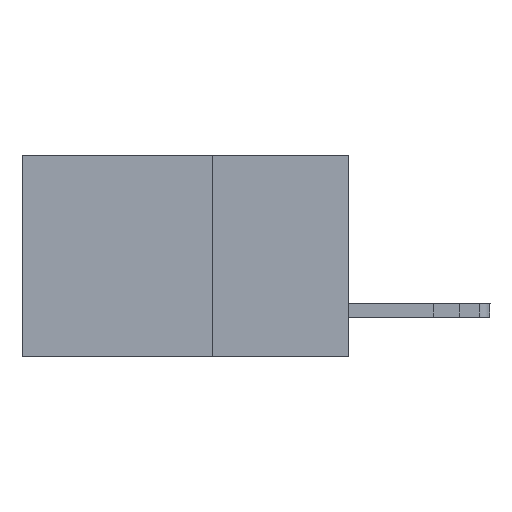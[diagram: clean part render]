
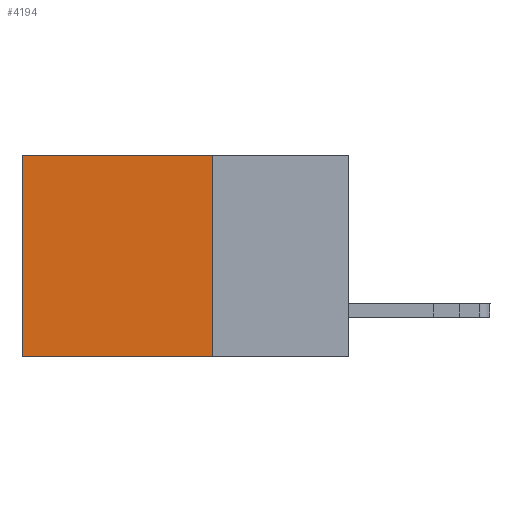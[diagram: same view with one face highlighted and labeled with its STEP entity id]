
A CAD part, left-side view. The second image highlights one B-rep face of the part: STEP entity #4194.
In plain terms, the highlighted planar face has unit normal (-1, 0, 0).
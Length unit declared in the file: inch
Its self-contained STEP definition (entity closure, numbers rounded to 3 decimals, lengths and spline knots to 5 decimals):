
#61 = ORIENTED_EDGE ( 'NONE', *, *, #4555, .F. ) ;
#358 = LINE ( 'NONE', #9970, #3960 ) ;
#395 = EDGE_CURVE ( 'NONE', #9664, #6442, #2372, .T. ) ;
#2223 = ORIENTED_EDGE ( 'NONE', *, *, #9491, .T. ) ;
#2327 = LINE ( 'NONE', #10978, #8749 ) ;
#2372 = LINE ( 'NONE', #5897, #4673 ) ;
#2373 = VERTEX_POINT ( 'NONE', #7644 ) ;
#2380 = VERTEX_POINT ( 'NONE', #3379 ) ;
#2879 = ORIENTED_EDGE ( 'NONE', *, *, #395, .T. ) ;
#2893 = CARTESIAN_POINT ( 'NONE',  ( 0.2615, 0.25, -0.37 ) ) ;
#3379 = CARTESIAN_POINT ( 'NONE',  ( 0.2615, 0.25, -0.37 ) ) ;
#3878 = DIRECTION ( 'NONE',  ( 0., 1., 0. ) ) ;
#3960 = VECTOR ( 'NONE', #3878, 39.37008 ) ;
#4194 = ADVANCED_FACE ( 'NONE', ( #10098 ), #9928, .F. ) ;
#4555 = EDGE_CURVE ( 'NONE', #2373, #2380, #8010, .T. ) ;
#4673 = VECTOR ( 'NONE', #10105, 39.37008 ) ;
#5897 = CARTESIAN_POINT ( 'NONE',  ( 0.2615, 0.6, -0.37 ) ) ;
#6170 = CARTESIAN_POINT ( 'NONE',  ( 0.2615, 0.25, -0.37 ) ) ;
#6442 = VERTEX_POINT ( 'NONE', #8867 ) ;
#7332 = DIRECTION ( 'NONE',  ( 0., 0., -1. ) ) ;
#7644 = CARTESIAN_POINT ( 'NONE',  ( 0.2615, 0.25, 0. ) ) ;
#8010 = LINE ( 'NONE', #6170, #9048 ) ;
#8375 = DIRECTION ( 'NONE',  ( 1., 0., 0. ) ) ;
#8749 = VECTOR ( 'NONE', #11143, 39.37008 ) ;
#8867 = CARTESIAN_POINT ( 'NONE',  ( 0.2615, 0.6, -0.37 ) ) ;
#9048 = VECTOR ( 'NONE', #9696, 39.37008 ) ;
#9153 = EDGE_CURVE ( 'NONE', #2380, #6442, #358, .T. ) ;
#9491 = EDGE_CURVE ( 'NONE', #2373, #9664, #2327, .T. ) ;
#9664 = VERTEX_POINT ( 'NONE', #11313 ) ;
#9696 = DIRECTION ( 'NONE',  ( 0., 0., -1. ) ) ;
#9928 = PLANE ( 'NONE',  #10076 ) ;
#9970 = CARTESIAN_POINT ( 'NONE',  ( 0.2615, 0.25, -0.37 ) ) ;
#10039 = ORIENTED_EDGE ( 'NONE', *, *, #9153, .F. ) ;
#10076 = AXIS2_PLACEMENT_3D ( 'NONE', #2893, #8375, #7332 ) ;
#10098 = FACE_OUTER_BOUND ( 'NONE', #11033, .T. ) ;
#10105 = DIRECTION ( 'NONE',  ( 0., 0., -1. ) ) ;
#10978 = CARTESIAN_POINT ( 'NONE',  ( 0.2615, 0.25, 0. ) ) ;
#11033 = EDGE_LOOP ( 'NONE', ( #2879, #10039, #61, #2223 ) ) ;
#11143 = DIRECTION ( 'NONE',  ( 0., 1., 0. ) ) ;
#11313 = CARTESIAN_POINT ( 'NONE',  ( 0.2615, 0.6, 0. ) ) ;
